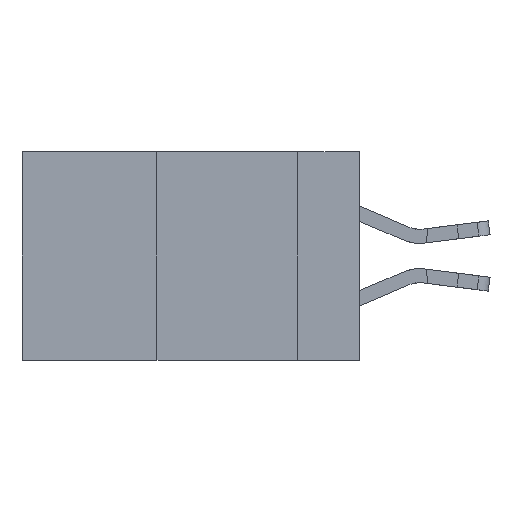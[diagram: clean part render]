
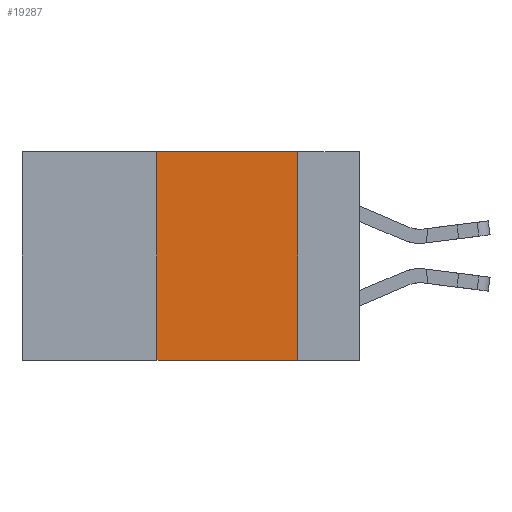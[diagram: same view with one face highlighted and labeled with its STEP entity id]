
A CAD part, left-side view. The second image highlights one B-rep face of the part: STEP entity #19287.
In plain terms, the highlighted planar face has unit normal (-1, 0, 0).
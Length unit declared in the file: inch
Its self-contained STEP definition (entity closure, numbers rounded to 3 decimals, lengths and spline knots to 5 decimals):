
#691 = DIRECTION ( 'NONE',  ( 0., 0., -1. ) ) ;
#712 = VECTOR ( 'NONE', #12778, 39.37008 ) ;
#863 = EDGE_LOOP ( 'NONE', ( #17930, #5705, #4445, #12294 ) ) ;
#1552 = CARTESIAN_POINT ( 'NONE',  ( 0., 0.36, 0. ) ) ;
#2071 = EDGE_CURVE ( 'NONE', #11439, #9809, #21050, .T. ) ;
#2112 = VERTEX_POINT ( 'NONE', #15079 ) ;
#2181 = DIRECTION ( 'NONE',  ( 0., -1., 0. ) ) ;
#3822 = PLANE ( 'NONE',  #8914 ) ;
#3835 = CARTESIAN_POINT ( 'NONE',  ( 0., 0.36, -0.37 ) ) ;
#4445 = ORIENTED_EDGE ( 'NONE', *, *, #2071, .F. ) ;
#4556 = DIRECTION ( 'NONE',  ( 0., 0., -1. ) ) ;
#4879 = VERTEX_POINT ( 'NONE', #14039 ) ;
#5359 = VECTOR ( 'NONE', #4556, 39.37008 ) ;
#5705 = ORIENTED_EDGE ( 'NONE', *, *, #8684, .F. ) ;
#6475 = CARTESIAN_POINT ( 'NONE',  ( 0., 0.11, 0. ) ) ;
#6877 = CARTESIAN_POINT ( 'NONE',  ( 0., 0.6, 0. ) ) ;
#7227 = CARTESIAN_POINT ( 'NONE',  ( 0., 0.36, 0. ) ) ;
#7640 = LINE ( 'NONE', #10649, #18548 ) ;
#8684 = EDGE_CURVE ( 'NONE', #9809, #2112, #8988, .T. ) ;
#8914 = AXIS2_PLACEMENT_3D ( 'NONE', #20041, #10297, #691 ) ;
#8988 = LINE ( 'NONE', #6877, #10763 ) ;
#9809 = VERTEX_POINT ( 'NONE', #7227 ) ;
#10297 = DIRECTION ( 'NONE',  ( 1., 0., 0. ) ) ;
#10649 = CARTESIAN_POINT ( 'NONE',  ( 0., 0.6, -0.37 ) ) ;
#10763 = VECTOR ( 'NONE', #2181, 39.37008 ) ;
#11439 = VERTEX_POINT ( 'NONE', #3835 ) ;
#11564 = FACE_OUTER_BOUND ( 'NONE', #863, .T. ) ;
#12294 = ORIENTED_EDGE ( 'NONE', *, *, #14160, .T. ) ;
#12778 = DIRECTION ( 'NONE',  ( 0., 0., 1. ) ) ;
#13304 = EDGE_CURVE ( 'NONE', #2112, #4879, #19121, .T. ) ;
#14039 = CARTESIAN_POINT ( 'NONE',  ( 0., 0.11, -0.37 ) ) ;
#14160 = EDGE_CURVE ( 'NONE', #11439, #4879, #7640, .T. ) ;
#15079 = CARTESIAN_POINT ( 'NONE',  ( 0., 0.11, 0. ) ) ;
#17180 = DIRECTION ( 'NONE',  ( 0., -1., 0. ) ) ;
#17930 = ORIENTED_EDGE ( 'NONE', *, *, #13304, .F. ) ;
#18548 = VECTOR ( 'NONE', #17180, 39.37008 ) ;
#19121 = LINE ( 'NONE', #6475, #5359 ) ;
#19287 = ADVANCED_FACE ( 'NONE', ( #11564 ), #3822, .F. ) ;
#20041 = CARTESIAN_POINT ( 'NONE',  ( 0., 0.6, 0. ) ) ;
#21050 = LINE ( 'NONE', #1552, #712 ) ;
